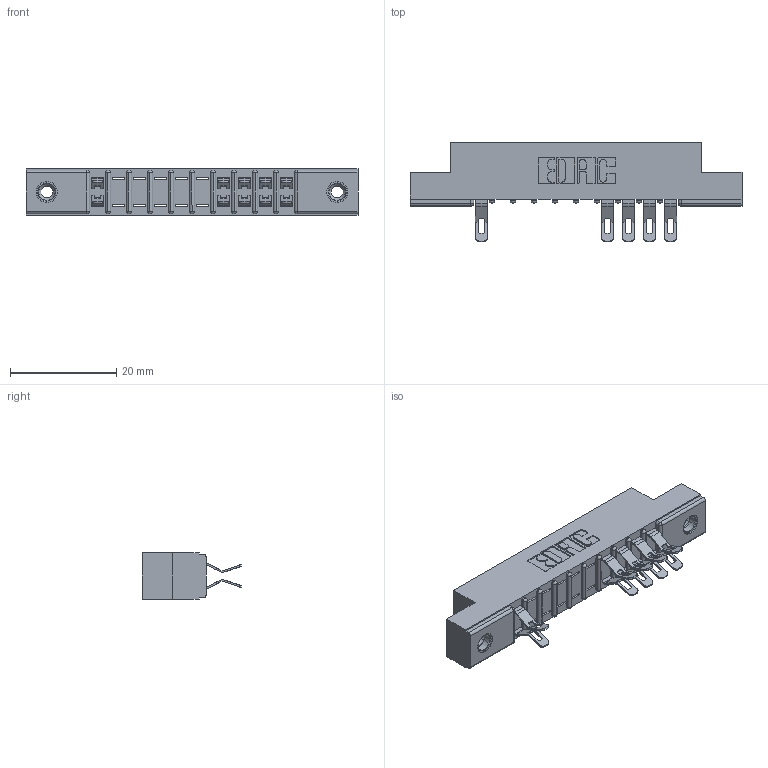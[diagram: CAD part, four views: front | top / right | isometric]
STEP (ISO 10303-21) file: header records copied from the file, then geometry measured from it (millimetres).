
FILE_DESCRIPTION (( 'STEP AP203' ), '1' );
FILE_NAME ('357-020-555-208.STEP', '2018-08-08T08:51:41', ( '' ), ( '' ), 'SwSTEP 2.0', 'SolidWorks 2016', '' );
FILE_SCHEMA (( 'CONFIG_CONTROL_DESIGN' ));
Length unit declared in the file: inch
Products named in the file (4): 357-020-555-208; 307 Part_.156 Dia Mounting Holes; 307-290-001_555; 345-250-001_345-250-003-102
Assembly tree (13 placements, depth 2):
  357-020-555-208
    307 Part_.156 Dia Mounting Holes
    307-290-001_555  x10
    345-250-001_345-250-003-102  x2
Bounding box: 62.64 x 18.75 x 8.71 mm (x, y, z)
Volume: 3992.2 mm3; surface area: 5847.1 mm2
Topology: 13 solids, 13 shells, 899 faces, 2589 edges, 1674 vertices
Faces by surface type: plane 502, cylinder 359, sphere 22, cone 12, torus 4
Entity records: 14240 total; most frequent: CARTESIAN_POINT 2371, ORIENTED_EDGE 2352, DIRECTION 2342, EDGE_CURVE 1176, VECTOR 876, LINE 876, VERTEX_POINT 762, AXIS2_PLACEMENT_3D 733
